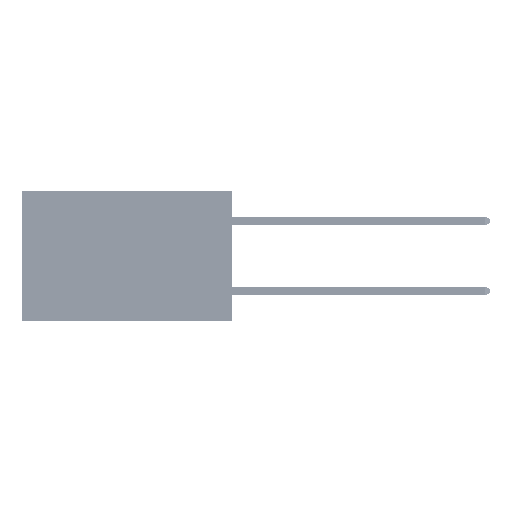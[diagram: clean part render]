
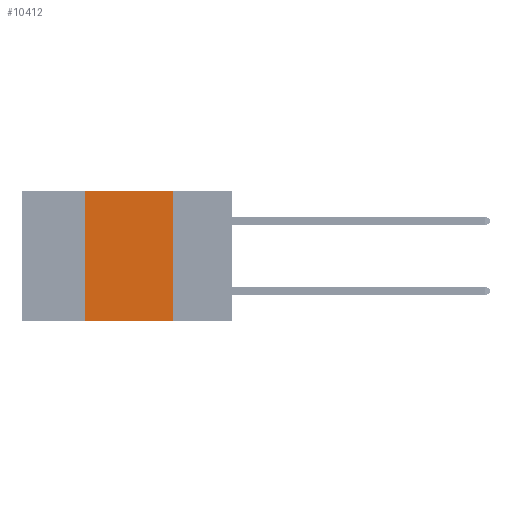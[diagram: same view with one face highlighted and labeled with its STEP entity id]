
A CAD part, left-side view. The second image highlights one B-rep face of the part: STEP entity #10412.
In plain terms, the highlighted planar face has unit normal (-1, 0, 0).
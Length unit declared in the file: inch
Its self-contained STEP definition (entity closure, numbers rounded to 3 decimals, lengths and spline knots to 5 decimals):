
#591 = CARTESIAN_POINT ( 'NONE',  ( 0., 0.6, 0. ) ) ;
#971 = DIRECTION ( 'NONE',  ( 1., 0., 0. ) ) ;
#3360 = FACE_OUTER_BOUND ( 'NONE', #45287, .T. ) ;
#4347 = DIRECTION ( 'NONE',  ( 0., 0., 1. ) ) ;
#4591 = PLANE ( 'NONE',  #35653 ) ;
#5253 = CARTESIAN_POINT ( 'NONE',  ( 0., 0.17, 0. ) ) ;
#6180 = VERTEX_POINT ( 'NONE', #9379 ) ;
#7749 = CARTESIAN_POINT ( 'NONE',  ( 0., 0.42, -0.37 ) ) ;
#9379 = CARTESIAN_POINT ( 'NONE',  ( 0., 0.17, 0. ) ) ;
#10302 = VERTEX_POINT ( 'NONE', #27264 ) ;
#10412 = ADVANCED_FACE ( 'NONE', ( #3360 ), #4591, .F. ) ;
#11595 = LINE ( 'NONE', #20248, #35165 ) ;
#13038 = ORIENTED_EDGE ( 'NONE', *, *, #43627, .F. ) ;
#15296 = ORIENTED_EDGE ( 'NONE', *, *, #44161, .T. ) ;
#18636 = CARTESIAN_POINT ( 'NONE',  ( 0., 0.6, -0.37 ) ) ;
#18974 = DIRECTION ( 'NONE',  ( 0., -1., 0. ) ) ;
#20248 = CARTESIAN_POINT ( 'NONE',  ( 0., 0.42, 0. ) ) ;
#22811 = VECTOR ( 'NONE', #47968, 39.37008 ) ;
#27264 = CARTESIAN_POINT ( 'NONE',  ( 0., 0.17, -0.37 ) ) ;
#29202 = CARTESIAN_POINT ( 'NONE',  ( 0., 0.42, 0. ) ) ;
#31922 = CARTESIAN_POINT ( 'NONE',  ( 0., 0.6, 0. ) ) ;
#32611 = DIRECTION ( 'NONE',  ( 0., 0., -1. ) ) ;
#32958 = ORIENTED_EDGE ( 'NONE', *, *, #47374, .F. ) ;
#34590 = VERTEX_POINT ( 'NONE', #7749 ) ;
#35165 = VECTOR ( 'NONE', #4347, 39.37008 ) ;
#35653 = AXIS2_PLACEMENT_3D ( 'NONE', #31922, #971, #32611 ) ;
#37003 = LINE ( 'NONE', #18636, #45034 ) ;
#40874 = DIRECTION ( 'NONE',  ( 0., 0., -1. ) ) ;
#42701 = LINE ( 'NONE', #5253, #50104 ) ;
#43398 = ORIENTED_EDGE ( 'NONE', *, *, #46388, .F. ) ;
#43627 = EDGE_CURVE ( 'NONE', #34590, #46881, #11595, .T. ) ;
#44161 = EDGE_CURVE ( 'NONE', #34590, #10302, #37003, .T. ) ;
#45034 = VECTOR ( 'NONE', #18974, 39.37008 ) ;
#45287 = EDGE_LOOP ( 'NONE', ( #43398, #32958, #13038, #15296 ) ) ;
#46388 = EDGE_CURVE ( 'NONE', #6180, #10302, #42701, .T. ) ;
#46881 = VERTEX_POINT ( 'NONE', #29202 ) ;
#47374 = EDGE_CURVE ( 'NONE', #46881, #6180, #50657, .T. ) ;
#47968 = DIRECTION ( 'NONE',  ( 0., -1., 0. ) ) ;
#50104 = VECTOR ( 'NONE', #40874, 39.37008 ) ;
#50657 = LINE ( 'NONE', #591, #22811 ) ;
